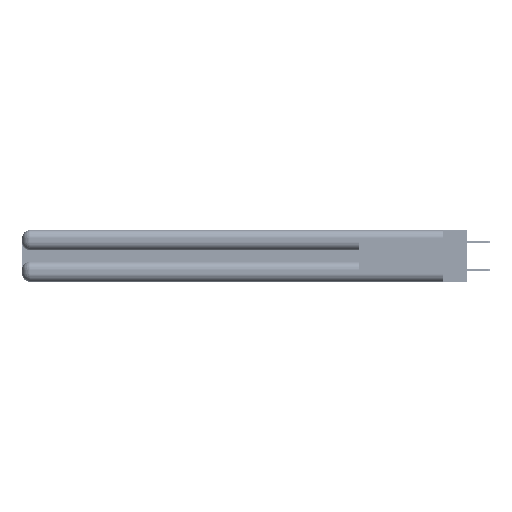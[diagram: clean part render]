
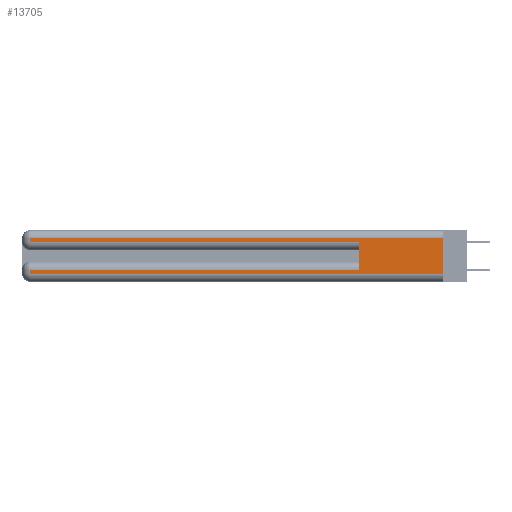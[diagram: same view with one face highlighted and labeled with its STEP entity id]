
A CAD part, left-side view. The second image highlights one B-rep face of the part: STEP entity #13705.
In plain terms, the highlighted planar face has unit normal (-1, 0, 0).
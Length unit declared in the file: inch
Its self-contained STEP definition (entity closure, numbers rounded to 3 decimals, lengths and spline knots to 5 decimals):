
#201 = EDGE_LOOP ( 'NONE', ( #2101, #15727, #20619, #27190, #42857, #32323, #27185, #17488 ) ) ;
#486 = VECTOR ( 'NONE', #3563, 39.37008 ) ;
#652 = VECTOR ( 'NONE', #4475, 39.37008 ) ;
#1308 = VECTOR ( 'NONE', #23833, 39.37008 ) ;
#1493 = DIRECTION ( 'NONE',  ( 1., 0., 0. ) ) ;
#2065 = VERTEX_POINT ( 'NONE', #34962 ) ;
#2101 = ORIENTED_EDGE ( 'NONE', *, *, #35515, .F. ) ;
#2522 = VERTEX_POINT ( 'NONE', #52312 ) ;
#2637 = LINE ( 'NONE', #32045, #1308 ) ;
#2945 = DIRECTION ( 'NONE',  ( 0., 0., 1. ) ) ;
#3563 = DIRECTION ( 'NONE',  ( 0., 0., -1. ) ) ;
#4475 = DIRECTION ( 'NONE',  ( 0., 0., -1. ) ) ;
#5225 = EDGE_CURVE ( 'NONE', #10097, #51066, #2637, .T. ) ;
#6955 = EDGE_CURVE ( 'NONE', #13848, #29008, #31231, .T. ) ;
#10097 = VERTEX_POINT ( 'NONE', #53764 ) ;
#10372 = VECTOR ( 'NONE', #34845, 39.37008 ) ;
#12068 = LINE ( 'NONE', #17791, #34217 ) ;
#12627 = DIRECTION ( 'NONE',  ( 0., -1., 0. ) ) ;
#13705 = ADVANCED_FACE ( 'NONE', ( #44232 ), #42988, .F. ) ;
#13829 = CARTESIAN_POINT ( 'NONE',  ( 0., 0., 0.37 ) ) ;
#13848 = VERTEX_POINT ( 'NONE', #19061 ) ;
#14390 = VECTOR ( 'NONE', #23202, 39.37008 ) ;
#15700 = LINE ( 'NONE', #43966, #14390 ) ;
#15727 = ORIENTED_EDGE ( 'NONE', *, *, #19457, .T. ) ;
#16941 = CARTESIAN_POINT ( 'NONE',  ( 0., 2.94, 0.37 ) ) ;
#17488 = ORIENTED_EDGE ( 'NONE', *, *, #31796, .T. ) ;
#17791 = CARTESIAN_POINT ( 'NONE',  ( 0., 0., 0.31 ) ) ;
#18707 = VECTOR ( 'NONE', #2945, 39.37008 ) ;
#19061 = CARTESIAN_POINT ( 'NONE',  ( 0., 0.6, 0.085 ) ) ;
#19457 = EDGE_CURVE ( 'NONE', #2065, #25661, #12068, .T. ) ;
#20619 = ORIENTED_EDGE ( 'NONE', *, *, #46726, .T. ) ;
#22797 = LINE ( 'NONE', #16941, #652 ) ;
#23202 = DIRECTION ( 'NONE',  ( 0., 0., -1. ) ) ;
#23719 = EDGE_CURVE ( 'NONE', #13848, #51066, #40903, .T. ) ;
#23833 = DIRECTION ( 'NONE',  ( 0., -1., 0. ) ) ;
#25661 = VERTEX_POINT ( 'NONE', #48292 ) ;
#26029 = VERTEX_POINT ( 'NONE', #30225 ) ;
#26667 = CARTESIAN_POINT ( 'NONE',  ( 0., 0., 0.085 ) ) ;
#27185 = ORIENTED_EDGE ( 'NONE', *, *, #42208, .T. ) ;
#27190 = ORIENTED_EDGE ( 'NONE', *, *, #5225, .T. ) ;
#28309 = CARTESIAN_POINT ( 'NONE',  ( 0., 2.94, 0.37 ) ) ;
#29008 = VERTEX_POINT ( 'NONE', #48073 ) ;
#30225 = CARTESIAN_POINT ( 'NONE',  ( 0., 0., 0.06 ) ) ;
#30630 = DIRECTION ( 'NONE',  ( 0., 0., -1. ) ) ;
#31231 = LINE ( 'NONE', #26667, #10372 ) ;
#31796 = EDGE_CURVE ( 'NONE', #2522, #26029, #36301, .T. ) ;
#32045 = CARTESIAN_POINT ( 'NONE',  ( 0., 0., 0.285 ) ) ;
#32323 = ORIENTED_EDGE ( 'NONE', *, *, #6955, .T. ) ;
#33737 = LINE ( 'NONE', #28309, #486 ) ;
#34217 = VECTOR ( 'NONE', #47029, 39.37008 ) ;
#34662 = CARTESIAN_POINT ( 'NONE',  ( 0., 0.6, 0.285 ) ) ;
#34845 = DIRECTION ( 'NONE',  ( 0., 1., 0. ) ) ;
#34962 = CARTESIAN_POINT ( 'NONE',  ( 0., 0., 0.31 ) ) ;
#35515 = EDGE_CURVE ( 'NONE', #2065, #26029, #15700, .T. ) ;
#36301 = LINE ( 'NONE', #45817, #48729 ) ;
#40903 = LINE ( 'NONE', #48650, #18707 ) ;
#42208 = EDGE_CURVE ( 'NONE', #29008, #2522, #33737, .T. ) ;
#42857 = ORIENTED_EDGE ( 'NONE', *, *, #23719, .F. ) ;
#42988 = PLANE ( 'NONE',  #47984 ) ;
#43966 = CARTESIAN_POINT ( 'NONE',  ( 0., 0., 0.37 ) ) ;
#44232 = FACE_OUTER_BOUND ( 'NONE', #201, .T. ) ;
#45817 = CARTESIAN_POINT ( 'NONE',  ( 0., 0., 0.06 ) ) ;
#46726 = EDGE_CURVE ( 'NONE', #25661, #10097, #22797, .T. ) ;
#47029 = DIRECTION ( 'NONE',  ( 0., 1., 0. ) ) ;
#47984 = AXIS2_PLACEMENT_3D ( 'NONE', #13829, #1493, #30630 ) ;
#48073 = CARTESIAN_POINT ( 'NONE',  ( 0., 2.94, 0.085 ) ) ;
#48292 = CARTESIAN_POINT ( 'NONE',  ( 0., 2.94, 0.31 ) ) ;
#48650 = CARTESIAN_POINT ( 'NONE',  ( 0., 0.6, 0.145 ) ) ;
#48729 = VECTOR ( 'NONE', #12627, 39.37008 ) ;
#51066 = VERTEX_POINT ( 'NONE', #34662 ) ;
#52312 = CARTESIAN_POINT ( 'NONE',  ( 0., 2.94, 0.06 ) ) ;
#53764 = CARTESIAN_POINT ( 'NONE',  ( 0., 2.94, 0.285 ) ) ;
